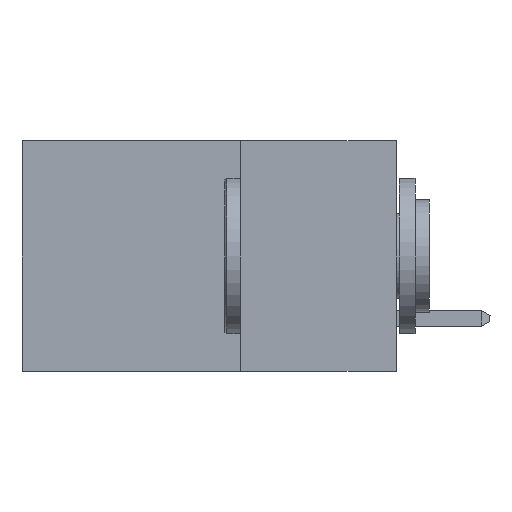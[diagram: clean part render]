
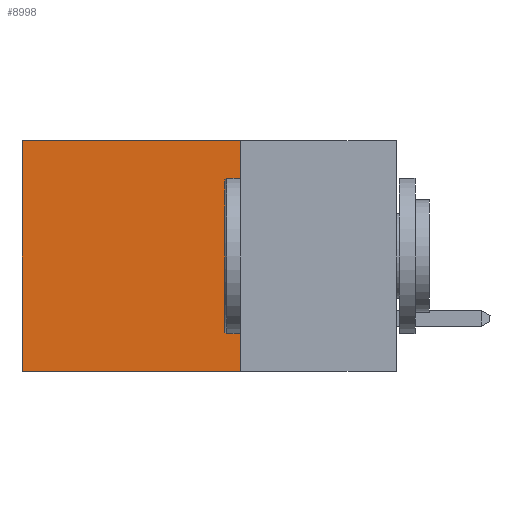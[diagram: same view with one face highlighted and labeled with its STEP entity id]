
A CAD part, left-side view. The second image highlights one B-rep face of the part: STEP entity #8998.
In plain terms, the highlighted planar face has unit normal (-1, 0, 0).
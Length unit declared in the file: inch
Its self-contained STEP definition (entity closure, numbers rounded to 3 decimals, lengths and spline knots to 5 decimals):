
#1117 = EDGE_CURVE ( 'NONE', #4515, #10268, #7697, .T. ) ;
#1173 = EDGE_LOOP ( 'NONE', ( #3533, #3466, #13066, #6349 ) ) ;
#1278 = CARTESIAN_POINT ( 'NONE',  ( 0.2615, 0.25, -0.37 ) ) ;
#1703 = VECTOR ( 'NONE', #5655, 39.37008 ) ;
#1828 = CARTESIAN_POINT ( 'NONE',  ( 0.2615, 0.6, -0.37 ) ) ;
#2071 = DIRECTION ( 'NONE',  ( 0., 1., 0. ) ) ;
#2193 = CARTESIAN_POINT ( 'NONE',  ( 0.2615, 0.25, -0.37 ) ) ;
#2405 = LINE ( 'NONE', #4123, #7385 ) ;
#2549 = CARTESIAN_POINT ( 'NONE',  ( 0.2615, 0.6, 0. ) ) ;
#3219 = DIRECTION ( 'NONE',  ( 0., 0., -1. ) ) ;
#3466 = ORIENTED_EDGE ( 'NONE', *, *, #1117, .F. ) ;
#3533 = ORIENTED_EDGE ( 'NONE', *, *, #10815, .T. ) ;
#4020 = CARTESIAN_POINT ( 'NONE',  ( 0.2615, 0.25, -0.37 ) ) ;
#4123 = CARTESIAN_POINT ( 'NONE',  ( 0.2615, 0.6, -0.37 ) ) ;
#4515 = VERTEX_POINT ( 'NONE', #12678 ) ;
#4617 = AXIS2_PLACEMENT_3D ( 'NONE', #4020, #11666, #11811 ) ;
#4821 = LINE ( 'NONE', #7122, #10046 ) ;
#5153 = VERTEX_POINT ( 'NONE', #5936 ) ;
#5566 = EDGE_CURVE ( 'NONE', #5153, #9247, #4821, .T. ) ;
#5655 = DIRECTION ( 'NONE',  ( 0., 0., -1. ) ) ;
#5936 = CARTESIAN_POINT ( 'NONE',  ( 0.2615, 0.25, 0. ) ) ;
#6349 = ORIENTED_EDGE ( 'NONE', *, *, #5566, .T. ) ;
#7122 = CARTESIAN_POINT ( 'NONE',  ( 0.2615, 0.25, 0. ) ) ;
#7385 = VECTOR ( 'NONE', #3219, 39.37008 ) ;
#7444 = FACE_OUTER_BOUND ( 'NONE', #1173, .T. ) ;
#7697 = LINE ( 'NONE', #2193, #9609 ) ;
#8079 = LINE ( 'NONE', #1278, #1703 ) ;
#8998 = ADVANCED_FACE ( 'NONE', ( #7444 ), #10762, .F. ) ;
#9247 = VERTEX_POINT ( 'NONE', #2549 ) ;
#9609 = VECTOR ( 'NONE', #2071, 39.37008 ) ;
#10046 = VECTOR ( 'NONE', #12860, 39.37008 ) ;
#10268 = VERTEX_POINT ( 'NONE', #1828 ) ;
#10762 = PLANE ( 'NONE',  #4617 ) ;
#10815 = EDGE_CURVE ( 'NONE', #9247, #10268, #2405, .T. ) ;
#11398 = EDGE_CURVE ( 'NONE', #5153, #4515, #8079, .T. ) ;
#11666 = DIRECTION ( 'NONE',  ( 1., 0., 0. ) ) ;
#11811 = DIRECTION ( 'NONE',  ( 0., 0., -1. ) ) ;
#12678 = CARTESIAN_POINT ( 'NONE',  ( 0.2615, 0.25, -0.37 ) ) ;
#12860 = DIRECTION ( 'NONE',  ( 0., 1., 0. ) ) ;
#13066 = ORIENTED_EDGE ( 'NONE', *, *, #11398, .F. ) ;
